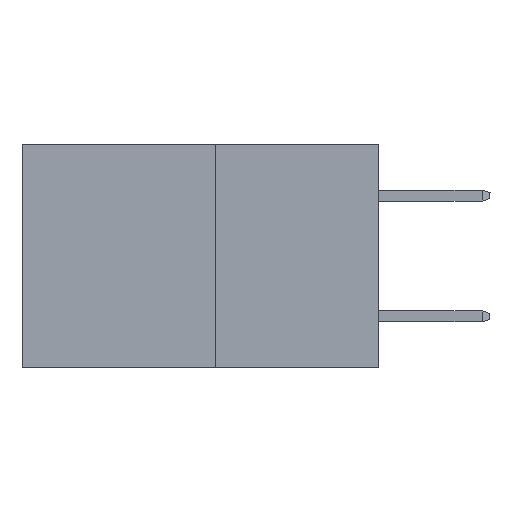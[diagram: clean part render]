
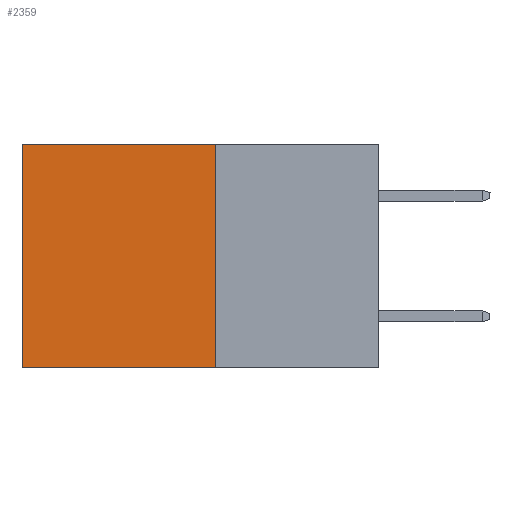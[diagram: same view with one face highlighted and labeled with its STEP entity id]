
A CAD part, left-side view. The second image highlights one B-rep face of the part: STEP entity #2359.
In plain terms, the highlighted planar face has unit normal (-1, 0, 0).
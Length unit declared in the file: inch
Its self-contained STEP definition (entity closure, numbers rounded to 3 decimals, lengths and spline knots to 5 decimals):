
#987 = CARTESIAN_POINT ( 'NONE',  ( 0.277, 0.27, -0.37 ) ) ;
#1026 = VERTEX_POINT ( 'NONE', #6863 ) ;
#1456 = LINE ( 'NONE', #987, #16094 ) ;
#2120 = CARTESIAN_POINT ( 'NONE',  ( 0.277, 0.27, -0.37 ) ) ;
#2292 = EDGE_LOOP ( 'NONE', ( #13066, #9244, #5605, #5131 ) ) ;
#2359 = ADVANCED_FACE ( 'NONE', ( #3981 ), #15322, .F. ) ;
#2639 = VERTEX_POINT ( 'NONE', #9313 ) ;
#2822 = CARTESIAN_POINT ( 'NONE',  ( 0.277, 0.59, -0.37 ) ) ;
#3570 = DIRECTION ( 'NONE',  ( 0., 1., 0. ) ) ;
#3981 = FACE_OUTER_BOUND ( 'NONE', #2292, .T. ) ;
#4303 = DIRECTION ( 'NONE',  ( 0., 0., -1. ) ) ;
#5131 = ORIENTED_EDGE ( 'NONE', *, *, #7241, .T. ) ;
#5605 = ORIENTED_EDGE ( 'NONE', *, *, #8853, .F. ) ;
#5935 = VECTOR ( 'NONE', #15045, 39.37008 ) ;
#6260 = VECTOR ( 'NONE', #4303, 39.37008 ) ;
#6863 = CARTESIAN_POINT ( 'NONE',  ( 0.277, 0.27, -0.37 ) ) ;
#7241 = EDGE_CURVE ( 'NONE', #2639, #8029, #17271, .T. ) ;
#7728 = VERTEX_POINT ( 'NONE', #10372 ) ;
#8029 = VERTEX_POINT ( 'NONE', #12476 ) ;
#8853 = EDGE_CURVE ( 'NONE', #2639, #1026, #1456, .T. ) ;
#9244 = ORIENTED_EDGE ( 'NONE', *, *, #10662, .F. ) ;
#9313 = CARTESIAN_POINT ( 'NONE',  ( 0.277, 0.27, 0. ) ) ;
#9318 = VECTOR ( 'NONE', #3570, 39.37008 ) ;
#9456 = DIRECTION ( 'NONE',  ( 0., 0., -1. ) ) ;
#9713 = CARTESIAN_POINT ( 'NONE',  ( 0.277, 0.27, -0.37 ) ) ;
#10372 = CARTESIAN_POINT ( 'NONE',  ( 0.277, 0.59, -0.37 ) ) ;
#10662 = EDGE_CURVE ( 'NONE', #1026, #7728, #16479, .T. ) ;
#12476 = CARTESIAN_POINT ( 'NONE',  ( 0.277, 0.59, 0. ) ) ;
#12579 = DIRECTION ( 'NONE',  ( 1., 0., 0. ) ) ;
#12597 = DIRECTION ( 'NONE',  ( 0., 0., -1. ) ) ;
#13066 = ORIENTED_EDGE ( 'NONE', *, *, #16001, .T. ) ;
#13651 = CARTESIAN_POINT ( 'NONE',  ( 0.277, 0.27, 0. ) ) ;
#14118 = AXIS2_PLACEMENT_3D ( 'NONE', #9713, #12579, #12597 ) ;
#15045 = DIRECTION ( 'NONE',  ( 0., 1., 0. ) ) ;
#15322 = PLANE ( 'NONE',  #14118 ) ;
#16001 = EDGE_CURVE ( 'NONE', #8029, #7728, #17599, .T. ) ;
#16094 = VECTOR ( 'NONE', #9456, 39.37008 ) ;
#16479 = LINE ( 'NONE', #2120, #9318 ) ;
#17271 = LINE ( 'NONE', #13651, #5935 ) ;
#17599 = LINE ( 'NONE', #2822, #6260 ) ;
